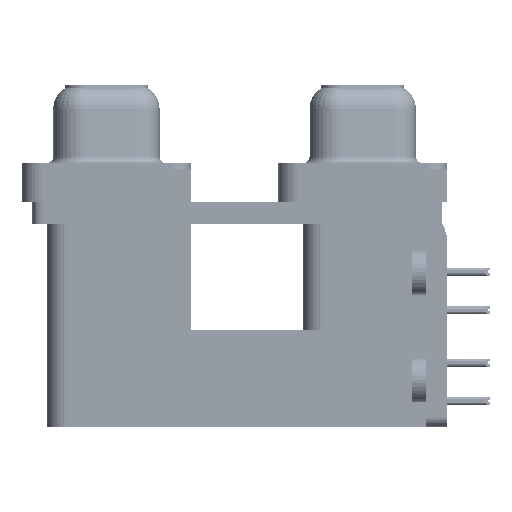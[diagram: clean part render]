
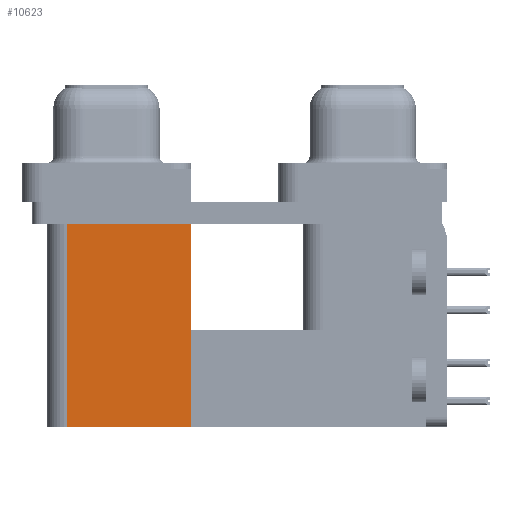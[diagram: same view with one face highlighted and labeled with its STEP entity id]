
A CAD part, left-side view. The second image highlights one B-rep face of the part: STEP entity #10623.
In plain terms, the highlighted planar face has unit normal (-1, 0, 0).
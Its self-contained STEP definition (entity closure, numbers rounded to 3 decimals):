
#1956 = CARTESIAN_POINT ( 'NONE',  ( 3.79, 12.775, -19.2 ) ) ;
#2960 = ORIENTED_EDGE ( 'NONE', *, *, #46537, .T. ) ;
#4715 = EDGE_CURVE ( 'NONE', #69908, #35104, #48631, .T. ) ;
#5498 = AXIS2_PLACEMENT_3D ( 'NONE', #10104, #33465, #50575 ) ;
#5840 = DIRECTION ( 'NONE',  ( 0., 1., 0. ) ) ;
#6934 = CARTESIAN_POINT ( 'NONE',  ( 3.79, 12.775, -19.2 ) ) ;
#8823 = LINE ( 'NONE', #19709, #66309 ) ;
#10104 = CARTESIAN_POINT ( 'NONE',  ( 3.79, 12.775, -19.2 ) ) ;
#10623 = ADVANCED_FACE ( 'NONE', ( #17737 ), #75429, .F. ) ;
#17737 = FACE_OUTER_BOUND ( 'NONE', #71947, .T. ) ;
#19488 = DIRECTION ( 'NONE',  ( 0., 0., 1. ) ) ;
#19709 = CARTESIAN_POINT ( 'NONE',  ( 3.79, 21.975, -19.2 ) ) ;
#19859 = DIRECTION ( 'NONE',  ( 0., 1., 0. ) ) ;
#20263 = LINE ( 'NONE', #1956, #76922 ) ;
#23780 = EDGE_CURVE ( 'NONE', #35104, #25366, #8823, .T. ) ;
#25366 = VERTEX_POINT ( 'NONE', #34044 ) ;
#26090 = LINE ( 'NONE', #55629, #32894 ) ;
#28607 = CARTESIAN_POINT ( 'NONE',  ( 3.79, 21.975, -19.2 ) ) ;
#32733 = VECTOR ( 'NONE', #5840, 1000. ) ;
#32894 = VECTOR ( 'NONE', #19859, 1000. ) ;
#33465 = DIRECTION ( 'NONE',  ( 1., 0., 0. ) ) ;
#34044 = CARTESIAN_POINT ( 'NONE',  ( 3.79, 21.975, -2.5 ) ) ;
#34366 = EDGE_CURVE ( 'NONE', #55375, #25366, #26090, .T. ) ;
#35104 = VERTEX_POINT ( 'NONE', #28607 ) ;
#38402 = DIRECTION ( 'NONE',  ( 0., 0., 1. ) ) ;
#43190 = CARTESIAN_POINT ( 'NONE',  ( 3.79, 12.775, -19.2 ) ) ;
#46537 = EDGE_CURVE ( 'NONE', #69908, #55375, #20263, .T. ) ;
#48631 = LINE ( 'NONE', #43190, #32733 ) ;
#48893 = ORIENTED_EDGE ( 'NONE', *, *, #23780, .F. ) ;
#50575 = DIRECTION ( 'NONE',  ( 0., 0., -1. ) ) ;
#55375 = VERTEX_POINT ( 'NONE', #71152 ) ;
#55499 = ORIENTED_EDGE ( 'NONE', *, *, #4715, .F. ) ;
#55629 = CARTESIAN_POINT ( 'NONE',  ( 3.79, 12.775, -2.5 ) ) ;
#66309 = VECTOR ( 'NONE', #38402, 1000. ) ;
#68842 = ORIENTED_EDGE ( 'NONE', *, *, #34366, .T. ) ;
#69908 = VERTEX_POINT ( 'NONE', #6934 ) ;
#71152 = CARTESIAN_POINT ( 'NONE',  ( 3.79, 12.775, -2.5 ) ) ;
#71947 = EDGE_LOOP ( 'NONE', ( #68842, #48893, #55499, #2960 ) ) ;
#75429 = PLANE ( 'NONE',  #5498 ) ;
#76922 = VECTOR ( 'NONE', #19488, 1000. ) ;
